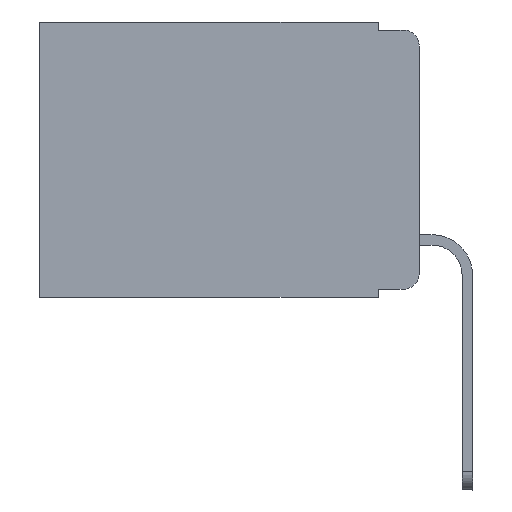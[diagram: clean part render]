
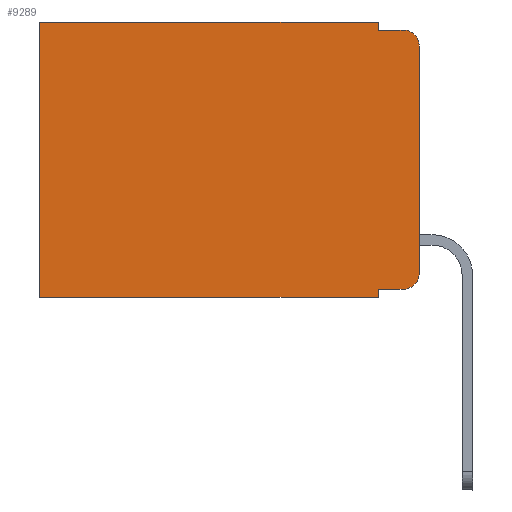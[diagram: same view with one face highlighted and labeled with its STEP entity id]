
A CAD part, left-side view. The second image highlights one B-rep face of the part: STEP entity #9289.
In plain terms, the highlighted planar face has unit normal (-1, 0, 0).
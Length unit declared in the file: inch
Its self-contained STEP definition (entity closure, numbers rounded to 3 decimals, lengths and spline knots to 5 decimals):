
#78 = ORIENTED_EDGE ( 'NONE', *, *, #98, .F. ) ;
#98 = EDGE_CURVE ( 'NONE', #11980, #15713, #830, .T. ) ;
#389 = EDGE_CURVE ( 'NONE', #11254, #13314, #12442, .T. ) ;
#688 = ORIENTED_EDGE ( 'NONE', *, *, #389, .T. ) ;
#700 = CARTESIAN_POINT ( 'NONE',  ( 0.298, 0., -0.313 ) ) ;
#830 = LINE ( 'NONE', #9409, #9352 ) ;
#894 = EDGE_CURVE ( 'NONE', #12223, #16109, #9615, .T. ) ;
#1048 = CARTESIAN_POINT ( 'NONE',  ( 0.298, 0.051, -0.01 ) ) ;
#1642 = DIRECTION ( 'NONE',  ( 0., 0., -1. ) ) ;
#2023 = PLANE ( 'NONE',  #11811 ) ;
#2651 = CARTESIAN_POINT ( 'NONE',  ( 0.298, 0.473, -0.343 ) ) ;
#2960 = ORIENTED_EDGE ( 'NONE', *, *, #10608, .T. ) ;
#3372 = VECTOR ( 'NONE', #12386, 39.37008 ) ;
#3705 = DIRECTION ( 'NONE',  ( 0., 0., -1. ) ) ;
#3816 = CARTESIAN_POINT ( 'NONE',  ( 0.298, 0., 0. ) ) ;
#3907 = VECTOR ( 'NONE', #7446, 39.37008 ) ;
#4001 = EDGE_CURVE ( 'NONE', #9304, #6211, #5230, .T. ) ;
#4090 = VECTOR ( 'NONE', #6423, 39.37008 ) ;
#4094 = EDGE_CURVE ( 'NONE', #15713, #16109, #5317, .T. ) ;
#4267 = CARTESIAN_POINT ( 'NONE',  ( 0.298, 0.051, -0.333 ) ) ;
#4353 = CARTESIAN_POINT ( 'NONE',  ( 0.298, 0.02, -0.01 ) ) ;
#4612 = LINE ( 'NONE', #4702, #15048 ) ;
#4677 = DIRECTION ( 'NONE',  ( -1., 0., 0. ) ) ;
#4702 = CARTESIAN_POINT ( 'NONE',  ( 0.298, 0.051, -0.01 ) ) ;
#4774 = CIRCLE ( 'NONE', #10371, 0.02 ) ;
#5142 = ORIENTED_EDGE ( 'NONE', *, *, #15376, .T. ) ;
#5230 = LINE ( 'NONE', #14805, #4090 ) ;
#5317 = LINE ( 'NONE', #6695, #9404 ) ;
#5414 = EDGE_LOOP ( 'NONE', ( #15773, #2960, #9485, #12416, #16862, #8924, #17425, #78, #5142, #688 ) ) ;
#5600 = LINE ( 'NONE', #15638, #3907 ) ;
#5836 = CARTESIAN_POINT ( 'NONE',  ( 0.298, 0.473, 0. ) ) ;
#5846 = CARTESIAN_POINT ( 'NONE',  ( 0.298, 0.051, -0.333 ) ) ;
#6073 = CARTESIAN_POINT ( 'NONE',  ( 0.298, 0.051, 0. ) ) ;
#6112 = CARTESIAN_POINT ( 'NONE',  ( 0.298, 0., -0.03 ) ) ;
#6211 = VERTEX_POINT ( 'NONE', #1048 ) ;
#6228 = EDGE_CURVE ( 'NONE', #14923, #13314, #14943, .T. ) ;
#6423 = DIRECTION ( 'NONE',  ( 0., 0., -1. ) ) ;
#6446 = DIRECTION ( 'NONE',  ( 0., 0., -1. ) ) ;
#6695 = CARTESIAN_POINT ( 'NONE',  ( 0.298, 0., -0.343 ) ) ;
#7423 = AXIS2_PLACEMENT_3D ( 'NONE', #14258, #4677, #1642 ) ;
#7446 = DIRECTION ( 'NONE',  ( 0., 1., 0. ) ) ;
#7644 = DIRECTION ( 'NONE',  ( 0., 0., -1. ) ) ;
#8924 = ORIENTED_EDGE ( 'NONE', *, *, #894, .T. ) ;
#9289 = ADVANCED_FACE ( 'NONE', ( #17589 ), #2023, .F. ) ;
#9304 = VERTEX_POINT ( 'NONE', #6073 ) ;
#9352 = VECTOR ( 'NONE', #6446, 39.37008 ) ;
#9404 = VECTOR ( 'NONE', #14893, 39.37008 ) ;
#9409 = CARTESIAN_POINT ( 'NONE',  ( 0.298, 0.051, 0. ) ) ;
#9471 = DIRECTION ( 'NONE',  ( 0., -1., 0. ) ) ;
#9485 = ORIENTED_EDGE ( 'NONE', *, *, #10438, .F. ) ;
#9615 = LINE ( 'NONE', #5836, #3372 ) ;
#9728 = CARTESIAN_POINT ( 'NONE',  ( 0.298, 0.473, 0. ) ) ;
#10371 = AXIS2_PLACEMENT_3D ( 'NONE', #16037, #16117, #3705 ) ;
#10438 = EDGE_CURVE ( 'NONE', #6211, #15506, #4612, .T. ) ;
#10608 = EDGE_CURVE ( 'NONE', #14923, #15506, #4774, .T. ) ;
#10808 = EDGE_CURVE ( 'NONE', #9304, #12223, #5600, .T. ) ;
#11254 = VERTEX_POINT ( 'NONE', #18218 ) ;
#11811 = AXIS2_PLACEMENT_3D ( 'NONE', #16112, #14639, #7644 ) ;
#11980 = VERTEX_POINT ( 'NONE', #5846 ) ;
#12209 = DIRECTION ( 'NONE',  ( 0., 0., -1. ) ) ;
#12223 = VERTEX_POINT ( 'NONE', #9728 ) ;
#12386 = DIRECTION ( 'NONE',  ( 0., 0., -1. ) ) ;
#12416 = ORIENTED_EDGE ( 'NONE', *, *, #4001, .F. ) ;
#12442 = CIRCLE ( 'NONE', #7423, 0.02 ) ;
#13314 = VERTEX_POINT ( 'NONE', #700 ) ;
#13581 = VECTOR ( 'NONE', #12209, 39.37008 ) ;
#14103 = DIRECTION ( 'NONE',  ( 0., -1., 0. ) ) ;
#14116 = LINE ( 'NONE', #4267, #16300 ) ;
#14258 = CARTESIAN_POINT ( 'NONE',  ( 0.298, 0.02, -0.313 ) ) ;
#14639 = DIRECTION ( 'NONE',  ( 1., 0., 0. ) ) ;
#14805 = CARTESIAN_POINT ( 'NONE',  ( 0.298, 0.051, 0. ) ) ;
#14893 = DIRECTION ( 'NONE',  ( 0., 1., 0. ) ) ;
#14923 = VERTEX_POINT ( 'NONE', #6112 ) ;
#14943 = LINE ( 'NONE', #3816, #13581 ) ;
#15048 = VECTOR ( 'NONE', #14103, 39.37008 ) ;
#15376 = EDGE_CURVE ( 'NONE', #11980, #11254, #14116, .T. ) ;
#15506 = VERTEX_POINT ( 'NONE', #4353 ) ;
#15638 = CARTESIAN_POINT ( 'NONE',  ( 0.298, 0., 0. ) ) ;
#15713 = VERTEX_POINT ( 'NONE', #17890 ) ;
#15773 = ORIENTED_EDGE ( 'NONE', *, *, #6228, .F. ) ;
#16037 = CARTESIAN_POINT ( 'NONE',  ( 0.298, 0.02, -0.03 ) ) ;
#16109 = VERTEX_POINT ( 'NONE', #2651 ) ;
#16112 = CARTESIAN_POINT ( 'NONE',  ( 0.298, 0., 0. ) ) ;
#16117 = DIRECTION ( 'NONE',  ( -1., 0., 0. ) ) ;
#16300 = VECTOR ( 'NONE', #9471, 39.37008 ) ;
#16862 = ORIENTED_EDGE ( 'NONE', *, *, #10808, .T. ) ;
#17425 = ORIENTED_EDGE ( 'NONE', *, *, #4094, .F. ) ;
#17589 = FACE_OUTER_BOUND ( 'NONE', #5414, .T. ) ;
#17890 = CARTESIAN_POINT ( 'NONE',  ( 0.298, 0.051, -0.343 ) ) ;
#18218 = CARTESIAN_POINT ( 'NONE',  ( 0.298, 0.02, -0.333 ) ) ;
